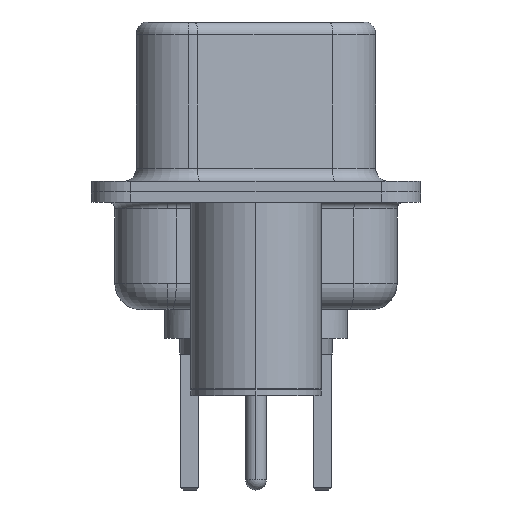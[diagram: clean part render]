
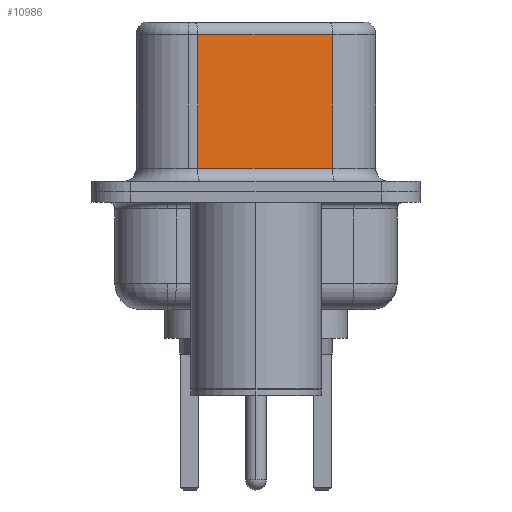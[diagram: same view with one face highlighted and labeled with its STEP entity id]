
A CAD part, left-side view. The second image highlights one B-rep face of the part: STEP entity #10986.
In plain terms, the highlighted planar face has unit normal (-0.985, -0.174, 0).
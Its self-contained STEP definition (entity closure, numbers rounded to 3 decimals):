
#70 = VECTOR ( 'NONE', #14273, 1000. ) ;
#1147 = DIRECTION ( 'NONE',  ( 0.174, -0.985, 0. ) ) ;
#1372 = ORIENTED_EDGE ( 'NONE', *, *, #12157, .T. ) ;
#1591 = LINE ( 'NONE', #16232, #7093 ) ;
#2148 = PLANE ( 'NONE',  #9540 ) ;
#2389 = LINE ( 'NONE', #15911, #6417 ) ;
#3164 = EDGE_CURVE ( 'NONE', #4836, #7919, #1591, .T. ) ;
#3960 = DIRECTION ( 'NONE',  ( 0., 0., -1. ) ) ;
#4808 = CARTESIAN_POINT ( 'NONE',  ( 3.675, 2.233, 6.52 ) ) ;
#4836 = VERTEX_POINT ( 'NONE', #11304 ) ;
#4881 = DIRECTION ( 'NONE',  ( -0.174, 0.985, 0. ) ) ;
#6417 = VECTOR ( 'NONE', #7801, 1000. ) ;
#6518 = VECTOR ( 'NONE', #1147, 1000. ) ;
#7093 = VECTOR ( 'NONE', #3960, 1000. ) ;
#7307 = LINE ( 'NONE', #4808, #70 ) ;
#7401 = CARTESIAN_POINT ( 'NONE',  ( 3.675, 2.233, 0.9 ) ) ;
#7801 = DIRECTION ( 'NONE',  ( -0.174, 0.985, 0. ) ) ;
#7919 = VERTEX_POINT ( 'NONE', #11186 ) ;
#9540 = AXIS2_PLACEMENT_3D ( 'NONE', #11647, #13009, #4881 ) ;
#9881 = ORIENTED_EDGE ( 'NONE', *, *, #16333, .T. ) ;
#9883 = ORIENTED_EDGE ( 'NONE', *, *, #15116, .T. ) ;
#10637 = CARTESIAN_POINT ( 'NONE',  ( 3.675, 2.233, 6.02 ) ) ;
#10656 = CARTESIAN_POINT ( 'NONE',  ( 4.585, -2.927, 0.9 ) ) ;
#10986 = ADVANCED_FACE ( 'NONE', ( #14165 ), #2148, .F. ) ;
#11186 = CARTESIAN_POINT ( 'NONE',  ( 4.585, -2.927, 0.9 ) ) ;
#11304 = CARTESIAN_POINT ( 'NONE',  ( 4.585, -2.927, 6.02 ) ) ;
#11647 = CARTESIAN_POINT ( 'NONE',  ( 4.585, -2.927, 6.52 ) ) ;
#11889 = VERTEX_POINT ( 'NONE', #7401 ) ;
#12157 = EDGE_CURVE ( 'NONE', #11889, #7919, #16492, .T. ) ;
#12755 = EDGE_LOOP ( 'NONE', ( #14751, #9881, #9883, #1372 ) ) ;
#13009 = DIRECTION ( 'NONE',  ( 0.985, 0.174, 0. ) ) ;
#14165 = FACE_OUTER_BOUND ( 'NONE', #12755, .T. ) ;
#14273 = DIRECTION ( 'NONE',  ( 0., 0., -1. ) ) ;
#14674 = VERTEX_POINT ( 'NONE', #10637 ) ;
#14751 = ORIENTED_EDGE ( 'NONE', *, *, #3164, .F. ) ;
#15116 = EDGE_CURVE ( 'NONE', #14674, #11889, #7307, .T. ) ;
#15911 = CARTESIAN_POINT ( 'NONE',  ( 4.585, -2.927, 6.02 ) ) ;
#16232 = CARTESIAN_POINT ( 'NONE',  ( 4.585, -2.927, 6.52 ) ) ;
#16333 = EDGE_CURVE ( 'NONE', #4836, #14674, #2389, .T. ) ;
#16492 = LINE ( 'NONE', #10656, #6518 ) ;
